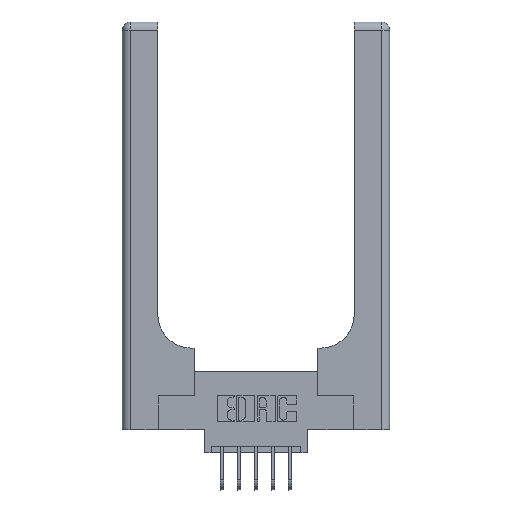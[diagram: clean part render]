
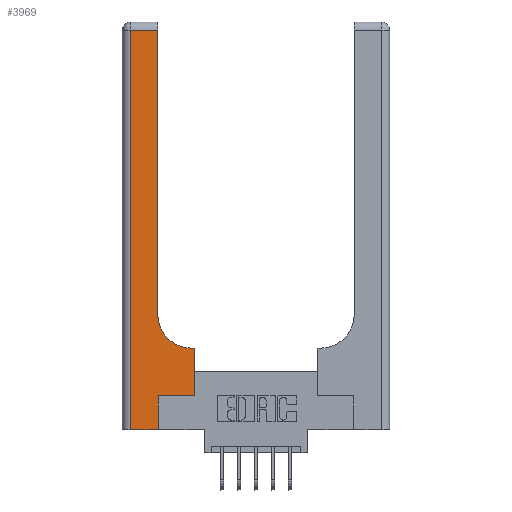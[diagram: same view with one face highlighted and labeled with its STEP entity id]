
A CAD part, top view. The second image highlights one B-rep face of the part: STEP entity #3969.
In plain terms, the highlighted planar face has unit normal (0, 0, 1).
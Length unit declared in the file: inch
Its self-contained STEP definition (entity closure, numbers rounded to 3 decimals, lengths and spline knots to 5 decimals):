
#485 = CARTESIAN_POINT ( 'NONE',  ( 0.528, 0.25, 0.37 ) ) ;
#543 = VECTOR ( 'NONE', #11792, 39.37008 ) ;
#627 = ORIENTED_EDGE ( 'NONE', *, *, #4953, .T. ) ;
#928 = VERTEX_POINT ( 'NONE', #2658 ) ;
#1750 = ORIENTED_EDGE ( 'NONE', *, *, #9361, .T. ) ;
#1947 = VERTEX_POINT ( 'NONE', #5657 ) ;
#1949 = DIRECTION ( 'NONE',  ( -1., 0., 0. ) ) ;
#2047 = LINE ( 'NONE', #13370, #543 ) ;
#2320 = DIRECTION ( 'NONE',  ( 1., 0., 0. ) ) ;
#2658 = CARTESIAN_POINT ( 'NONE',  ( 0.528, 0.6, 0.37 ) ) ;
#2794 = ORIENTED_EDGE ( 'NONE', *, *, #9420, .T. ) ;
#3155 = LINE ( 'NONE', #14318, #3578 ) ;
#3537 = CARTESIAN_POINT ( 'NONE',  ( 0.06, 0., 0.37 ) ) ;
#3578 = VECTOR ( 'NONE', #1949, 39.37008 ) ;
#3827 = AXIS2_PLACEMENT_3D ( 'NONE', #7344, #11029, #2320 ) ;
#3885 = VECTOR ( 'NONE', #5538, 39.37008 ) ;
#3899 = VERTEX_POINT ( 'NONE', #485 ) ;
#3969 = ADVANCED_FACE ( 'NONE', ( #7925 ), #11675, .F. ) ;
#4057 = CARTESIAN_POINT ( 'NONE',  ( 0.26, 0.85, 0.37 ) ) ;
#4091 = VECTOR ( 'NONE', #13342, 39.37008 ) ;
#4290 = DIRECTION ( 'NONE',  ( -1., 0., 0. ) ) ;
#4369 = DIRECTION ( 'NONE',  ( 1., 0., 0. ) ) ;
#4396 = VERTEX_POINT ( 'NONE', #12993 ) ;
#4649 = LINE ( 'NONE', #8542, #4091 ) ;
#4953 = EDGE_CURVE ( 'NONE', #3899, #928, #15420, .T. ) ;
#5373 = ORIENTED_EDGE ( 'NONE', *, *, #8257, .T. ) ;
#5391 = EDGE_LOOP ( 'NONE', ( #7449, #14811, #15627, #6807, #2794, #7395, #627, #5373, #1750 ) ) ;
#5538 = DIRECTION ( 'NONE',  ( 0., 1., 0. ) ) ;
#5617 = DIRECTION ( 'NONE',  ( 0., 0., -1. ) ) ;
#5623 = CARTESIAN_POINT ( 'NONE',  ( 0.528, 0.25, 0.37 ) ) ;
#5657 = CARTESIAN_POINT ( 'NONE',  ( 0.265, 0.25, 0.37 ) ) ;
#5804 = LINE ( 'NONE', #8027, #11479 ) ;
#6029 = EDGE_CURVE ( 'NONE', #12221, #9018, #13031, .T. ) ;
#6807 = ORIENTED_EDGE ( 'NONE', *, *, #6029, .T. ) ;
#7067 = CARTESIAN_POINT ( 'NONE',  ( 0.06, 3., 0.37 ) ) ;
#7344 = CARTESIAN_POINT ( 'NONE',  ( 0.51, 0.85, 0.37 ) ) ;
#7395 = ORIENTED_EDGE ( 'NONE', *, *, #8462, .T. ) ;
#7449 = ORIENTED_EDGE ( 'NONE', *, *, #13002, .T. ) ;
#7925 = FACE_OUTER_BOUND ( 'NONE', #5391, .T. ) ;
#8027 = CARTESIAN_POINT ( 'NONE',  ( 0.265, 0.25, 0.37 ) ) ;
#8257 = EDGE_CURVE ( 'NONE', #928, #14158, #8994, .T. ) ;
#8433 = AXIS2_PLACEMENT_3D ( 'NONE', #9048, #5617, #13918 ) ;
#8462 = EDGE_CURVE ( 'NONE', #1947, #3899, #5804, .T. ) ;
#8542 = CARTESIAN_POINT ( 'NONE',  ( 0.265, 0., 0.37 ) ) ;
#8544 = CARTESIAN_POINT ( 'NONE',  ( 0.51, 0.6, 0.37 ) ) ;
#8858 = EDGE_CURVE ( 'NONE', #15265, #4396, #3155, .T. ) ;
#8912 = CARTESIAN_POINT ( 'NONE',  ( 0.26, 0.6, 0.37 ) ) ;
#8994 = LINE ( 'NONE', #8912, #10695 ) ;
#9018 = VERTEX_POINT ( 'NONE', #13280 ) ;
#9048 = CARTESIAN_POINT ( 'NONE',  ( 0., 3., 0.37 ) ) ;
#9361 = EDGE_CURVE ( 'NONE', #14158, #12855, #9948, .T. ) ;
#9420 = EDGE_CURVE ( 'NONE', #9018, #1947, #4649, .T. ) ;
#9948 = CIRCLE ( 'NONE', #3827, 0.25 ) ;
#9990 = CARTESIAN_POINT ( 'NONE',  ( 0.26, 2.94, 0.37 ) ) ;
#10461 = VECTOR ( 'NONE', #15425, 39.37008 ) ;
#10584 = LINE ( 'NONE', #7067, #10461 ) ;
#10591 = EDGE_CURVE ( 'NONE', #4396, #12221, #10584, .T. ) ;
#10695 = VECTOR ( 'NONE', #4290, 39.37008 ) ;
#11029 = DIRECTION ( 'NONE',  ( 0., 0., -1. ) ) ;
#11479 = VECTOR ( 'NONE', #4369, 39.37008 ) ;
#11675 = PLANE ( 'NONE',  #8433 ) ;
#11792 = DIRECTION ( 'NONE',  ( 0., 1., 0. ) ) ;
#12221 = VERTEX_POINT ( 'NONE', #3537 ) ;
#12855 = VERTEX_POINT ( 'NONE', #4057 ) ;
#12993 = CARTESIAN_POINT ( 'NONE',  ( 0.06, 2.94, 0.37 ) ) ;
#13002 = EDGE_CURVE ( 'NONE', #12855, #15265, #2047, .T. ) ;
#13031 = LINE ( 'NONE', #15491, #15469 ) ;
#13280 = CARTESIAN_POINT ( 'NONE',  ( 0.265, 0., 0.37 ) ) ;
#13342 = DIRECTION ( 'NONE',  ( 0., 1., 0. ) ) ;
#13370 = CARTESIAN_POINT ( 'NONE',  ( 0.26, 3., 0.37 ) ) ;
#13918 = DIRECTION ( 'NONE',  ( -1., 0., 0. ) ) ;
#14158 = VERTEX_POINT ( 'NONE', #8544 ) ;
#14311 = DIRECTION ( 'NONE',  ( 1., 0., 0. ) ) ;
#14318 = CARTESIAN_POINT ( 'NONE',  ( 0., 2.94, 0.37 ) ) ;
#14811 = ORIENTED_EDGE ( 'NONE', *, *, #8858, .T. ) ;
#15265 = VERTEX_POINT ( 'NONE', #9990 ) ;
#15420 = LINE ( 'NONE', #5623, #3885 ) ;
#15425 = DIRECTION ( 'NONE',  ( 0., -1., 0. ) ) ;
#15469 = VECTOR ( 'NONE', #14311, 39.37008 ) ;
#15491 = CARTESIAN_POINT ( 'NONE',  ( 0., 0., 0.37 ) ) ;
#15627 = ORIENTED_EDGE ( 'NONE', *, *, #10591, .T. ) ;
